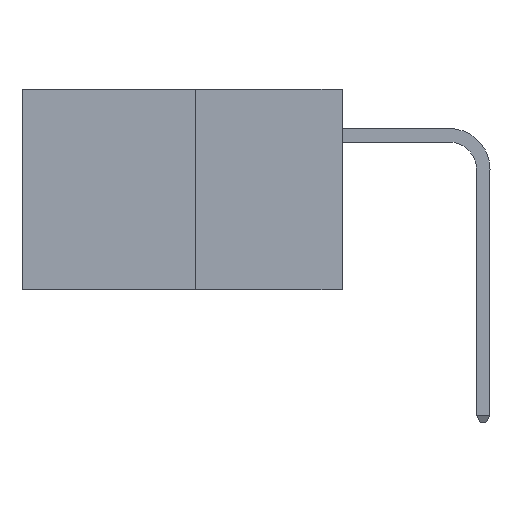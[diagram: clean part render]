
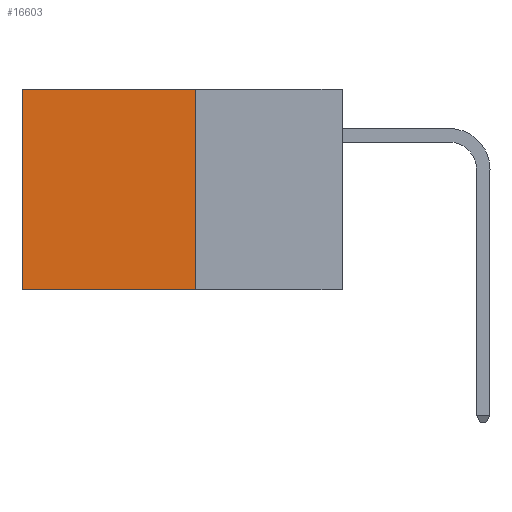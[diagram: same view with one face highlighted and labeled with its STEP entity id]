
A CAD part, left-side view. The second image highlights one B-rep face of the part: STEP entity #16603.
In plain terms, the highlighted planar face has unit normal (-1, 0, 0).
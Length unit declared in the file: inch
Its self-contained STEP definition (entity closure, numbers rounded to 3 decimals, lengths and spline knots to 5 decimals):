
#1592 = ORIENTED_EDGE ( 'NONE', *, *, #10513, .F. ) ;
#1623 = DIRECTION ( 'NONE',  ( 0., 1., 0. ) ) ;
#2362 = VERTEX_POINT ( 'NONE', #13363 ) ;
#2547 = DIRECTION ( 'NONE',  ( 1., 0., 0. ) ) ;
#2728 = LINE ( 'NONE', #11205, #15465 ) ;
#3983 = AXIS2_PLACEMENT_3D ( 'NONE', #13913, #2547, #15788 ) ;
#3987 = LINE ( 'NONE', #18272, #23422 ) ;
#6588 = CARTESIAN_POINT ( 'NONE',  ( 0.277, 0.27, -0.37 ) ) ;
#7266 = ORIENTED_EDGE ( 'NONE', *, *, #9285, .T. ) ;
#7340 = ORIENTED_EDGE ( 'NONE', *, *, #16927, .T. ) ;
#8828 = CARTESIAN_POINT ( 'NONE',  ( 0.277, 0.59, -0.37 ) ) ;
#9285 = EDGE_CURVE ( 'NONE', #2362, #17468, #2728, .T. ) ;
#10513 = EDGE_CURVE ( 'NONE', #13373, #12128, #3987, .T. ) ;
#10807 = DIRECTION ( 'NONE',  ( 0., 0., -1. ) ) ;
#10819 = CARTESIAN_POINT ( 'NONE',  ( 0.277, 0.27, -0.37 ) ) ;
#11163 = LINE ( 'NONE', #22318, #19971 ) ;
#11205 = CARTESIAN_POINT ( 'NONE',  ( 0.277, 0.59, -0.37 ) ) ;
#12040 = PLANE ( 'NONE',  #3983 ) ;
#12128 = VERTEX_POINT ( 'NONE', #10819 ) ;
#12585 = CARTESIAN_POINT ( 'NONE',  ( 0.277, 0.27, 0. ) ) ;
#13363 = CARTESIAN_POINT ( 'NONE',  ( 0.277, 0.59, 0. ) ) ;
#13373 = VERTEX_POINT ( 'NONE', #12585 ) ;
#13913 = CARTESIAN_POINT ( 'NONE',  ( 0.277, 0.27, -0.37 ) ) ;
#15071 = EDGE_LOOP ( 'NONE', ( #7266, #19931, #1592, #7340 ) ) ;
#15150 = VECTOR ( 'NONE', #17801, 39.37008 ) ;
#15465 = VECTOR ( 'NONE', #22403, 39.37008 ) ;
#15788 = DIRECTION ( 'NONE',  ( 0., 0., -1. ) ) ;
#16603 = ADVANCED_FACE ( 'NONE', ( #18204 ), #12040, .F. ) ;
#16927 = EDGE_CURVE ( 'NONE', #13373, #2362, #11163, .T. ) ;
#17468 = VERTEX_POINT ( 'NONE', #8828 ) ;
#17801 = DIRECTION ( 'NONE',  ( 0., 1., 0. ) ) ;
#18204 = FACE_OUTER_BOUND ( 'NONE', #15071, .T. ) ;
#18272 = CARTESIAN_POINT ( 'NONE',  ( 0.277, 0.27, -0.37 ) ) ;
#19931 = ORIENTED_EDGE ( 'NONE', *, *, #23581, .F. ) ;
#19971 = VECTOR ( 'NONE', #1623, 39.37008 ) ;
#22318 = CARTESIAN_POINT ( 'NONE',  ( 0.277, 0.27, 0. ) ) ;
#22403 = DIRECTION ( 'NONE',  ( 0., 0., -1. ) ) ;
#23422 = VECTOR ( 'NONE', #10807, 39.37008 ) ;
#23581 = EDGE_CURVE ( 'NONE', #12128, #17468, #23877, .T. ) ;
#23877 = LINE ( 'NONE', #6588, #15150 ) ;
